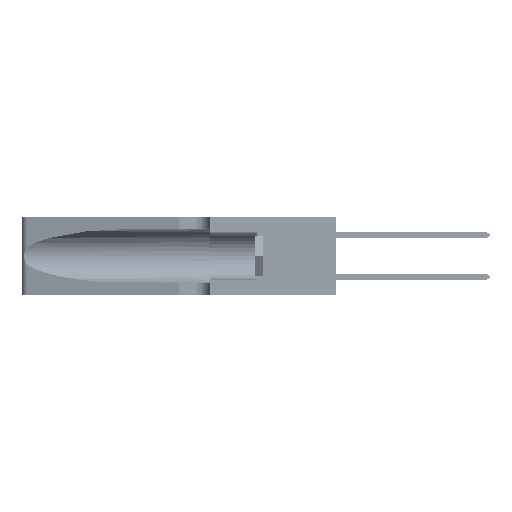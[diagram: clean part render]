
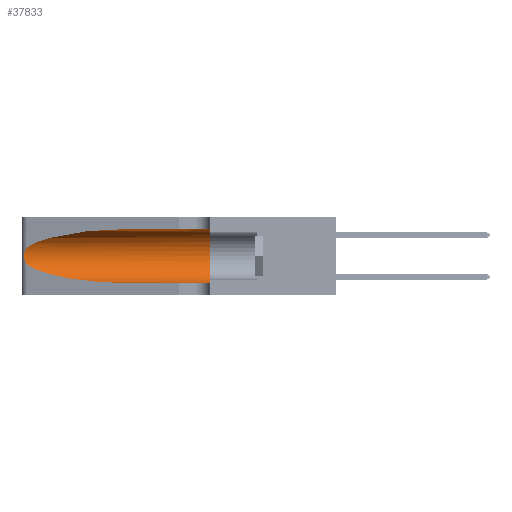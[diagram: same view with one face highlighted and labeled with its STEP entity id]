
A CAD part, left-side view. The second image highlights one B-rep face of the part: STEP entity #37833.
In plain terms, the highlighted cylindrical face has radius 3.308 mm (diameter 6.617 mm), a partial arc.
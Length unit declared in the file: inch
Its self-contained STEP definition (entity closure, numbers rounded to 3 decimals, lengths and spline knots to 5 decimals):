
#127 = CARTESIAN_POINT ( 'NONE',  ( 0.1305, 0.35, 0.185 ) ) ;
#399 = DIRECTION ( 'NONE',  ( 0., 0., -1. ) ) ;
#615 = CARTESIAN_POINT ( 'NONE',  ( 0.25639, 1.23186, 0.15144 ) ) ;
#1072 = ORIENTED_EDGE ( 'NONE', *, *, #36134, .T. ) ;
#2564 = ORIENTED_EDGE ( 'NONE', *, *, #10822, .T. ) ;
#3224 = LINE ( 'NONE', #31769, #21504 ) ;
#4847 = EDGE_LOOP ( 'NONE', ( #1072, #2564, #7027, #9130, #8624, #18576 ) ) ;
#6665 = EDGE_CURVE ( 'NONE', #41783, #29272, #3224, .T. ) ;
#7027 = ORIENTED_EDGE ( 'NONE', *, *, #41073, .T. ) ;
#7701 = CARTESIAN_POINT ( 'NONE',  ( 0.25555, 1.22993, 0.14849 ) ) ;
#7929 = CARTESIAN_POINT ( 'NONE',  ( 0.25487, 1.22718, 0.14631 ) ) ;
#8624 = ORIENTED_EDGE ( 'NONE', *, *, #37200, .F. ) ;
#9105 =( BOUNDED_CURVE ( )  B_SPLINE_CURVE ( 3, ( #7929, #34101, #14827, #41223 ),
 .UNSPECIFIED., .F., .F. ) 
 B_SPLINE_CURVE_WITH_KNOTS ( ( 4, 4 ),
 ( 3.44316, 4.71239 ),
 .UNSPECIFIED. ) 
 CURVE ( )  GEOMETRIC_REPRESENTATION_ITEM ( )  RATIONAL_B_SPLINE_CURVE ( ( 1., 0.87, 0.87, 1. ) ) 
 REPRESENTATION_ITEM ( '' )  );
#9130 = ORIENTED_EDGE ( 'NONE', *, *, #43528, .T. ) ;
#10653 = CARTESIAN_POINT ( 'NONE',  ( 0.25487, 1.22718, 0.22369 ) ) ;
#10822 = EDGE_CURVE ( 'NONE', #26432, #28056, #36006, .T. ) ;
#11378 = FACE_OUTER_BOUND ( 'NONE', #4847, .T. ) ;
#12547 = CYLINDRICAL_SURFACE ( 'NONE', #44460, 0.13025 ) ;
#14827 = CARTESIAN_POINT ( 'NONE',  ( 0.18966, 0.96281, 0.05475 ) ) ;
#15908 = CARTESIAN_POINT ( 'NONE',  ( 0.1305, 0.35, 0.31525 ) ) ;
#16165 = CARTESIAN_POINT ( 'NONE',  ( 0.25487, 1.22718, 0.14631 ) ) ;
#18576 = ORIENTED_EDGE ( 'NONE', *, *, #6665, .F. ) ;
#21504 = VECTOR ( 'NONE', #27485, 39.37008 ) ;
#21630 = VECTOR ( 'NONE', #29426, 39.37008 ) ;
#22163 = CARTESIAN_POINT ( 'NONE',  ( 0.25555, 1.22994, 0.2215 ) ) ;
#22607 = CIRCLE ( 'NONE', #30715, 0.13025 ) ;
#22977 = CARTESIAN_POINT ( 'NONE',  ( 0.25789, 1.23486, 0.15765 ) ) ;
#23130 = CARTESIAN_POINT ( 'NONE',  ( 0.25856, 1.23593, 0.16098 ) ) ;
#24032 = CARTESIAN_POINT ( 'NONE',  ( 0.2373, 1.15595, 0.28018 ) ) ;
#26219 = DIRECTION ( 'NONE',  ( 0., -1., 0. ) ) ;
#26238 = CARTESIAN_POINT ( 'NONE',  ( 0.1305, 0.35, 0.05475 ) ) ;
#26432 = VERTEX_POINT ( 'NONE', #33419 ) ;
#26607 = CARTESIAN_POINT ( 'NONE',  ( 0.26017, 1.23833, 0.17102 ) ) ;
#26736 = DIRECTION ( 'NONE',  ( 0., 0., 1. ) ) ;
#27485 = DIRECTION ( 'NONE',  ( 0., -1., 0. ) ) ;
#28056 = VERTEX_POINT ( 'NONE', #16165 ) ;
#29272 = VERTEX_POINT ( 'NONE', #15908 ) ;
#29426 = DIRECTION ( 'NONE',  ( 0., -1., 0. ) ) ;
#30715 = AXIS2_PLACEMENT_3D ( 'NONE', #127, #48725, #26736 ) ;
#31642 = LINE ( 'NONE', #48757, #21630 ) ;
#31769 = CARTESIAN_POINT ( 'NONE',  ( 0.1305, 1.61858, 0.31525 ) ) ;
#33419 = CARTESIAN_POINT ( 'NONE',  ( 0.25487, 1.22718, 0.22369 ) ) ;
#34101 = CARTESIAN_POINT ( 'NONE',  ( 0.2373, 1.15595, 0.08982 ) ) ;
#34506 = CARTESIAN_POINT ( 'NONE',  ( 0.25487, 1.22718, 0.14631 ) ) ;
#35426 = CARTESIAN_POINT ( 'NONE',  ( 0.25487, 1.22718, 0.22369 ) ) ;
#36006 = B_SPLINE_CURVE_WITH_KNOTS ( 'NONE', 3,
 ( #10653, #22163, #37004, #44639, #48439, #42126, #41477, #45777, #26607, #23130, #22977, #615, #7701, #34506 ),
 .UNSPECIFIED., .F., .F.,
 ( 4, 2, 2, 2, 2, 2, 4 ),
 ( 0., 0.00027, 0.00053, 0.00107, 0.0016, 0.00187, 0.00214 ),
 .UNSPECIFIED. ) ;
#36134 = EDGE_CURVE ( 'NONE', #41783, #26432, #43285, .T. ) ;
#37004 = CARTESIAN_POINT ( 'NONE',  ( 0.25639, 1.23184, 0.21858 ) ) ;
#37200 = EDGE_CURVE ( 'NONE', #29272, #40285, #22607, .T. ) ;
#37833 = ADVANCED_FACE ( 'NONE', ( #11378 ), #12547, .F. ) ;
#38315 = CARTESIAN_POINT ( 'NONE',  ( 0.1305, 0.72297, 0.31525 ) ) ;
#39038 = CARTESIAN_POINT ( 'NONE',  ( 0.1305, 0.72297, 0.31525 ) ) ;
#40285 = VERTEX_POINT ( 'NONE', #26238 ) ;
#41073 = EDGE_CURVE ( 'NONE', #28056, #47740, #9105, .T. ) ;
#41223 = CARTESIAN_POINT ( 'NONE',  ( 0.1305, 0.72297, 0.05475 ) ) ;
#41477 = CARTESIAN_POINT ( 'NONE',  ( 0.26075, 1.23896, 0.19203 ) ) ;
#41783 = VERTEX_POINT ( 'NONE', #38315 ) ;
#42126 = CARTESIAN_POINT ( 'NONE',  ( 0.26018, 1.23835, 0.19895 ) ) ;
#42543 = CARTESIAN_POINT ( 'NONE',  ( 0.1305, 0.72297, 0.05475 ) ) ;
#43285 =( BOUNDED_CURVE ( )  B_SPLINE_CURVE ( 3, ( #39038, #46681, #24032, #35426 ),
 .UNSPECIFIED., .F., .F. ) 
 B_SPLINE_CURVE_WITH_KNOTS ( ( 4, 4 ),
 ( 1.5708, 2.84003 ),
 .UNSPECIFIED. ) 
 CURVE ( )  GEOMETRIC_REPRESENTATION_ITEM ( )  RATIONAL_B_SPLINE_CURVE ( ( 1., 0.87, 0.87, 1. ) ) 
 REPRESENTATION_ITEM ( '' )  );
#43528 = EDGE_CURVE ( 'NONE', #47740, #40285, #31642, .T. ) ;
#44460 = AXIS2_PLACEMENT_3D ( 'NONE', #45563, #26219, #399 ) ;
#44639 = CARTESIAN_POINT ( 'NONE',  ( 0.25787, 1.23484, 0.2124 ) ) ;
#45563 = CARTESIAN_POINT ( 'NONE',  ( 0.1305, 1.61858, 0.185 ) ) ;
#45777 = CARTESIAN_POINT ( 'NONE',  ( 0.26075, 1.23896, 0.178 ) ) ;
#46681 = CARTESIAN_POINT ( 'NONE',  ( 0.18966, 0.96281, 0.31525 ) ) ;
#47740 = VERTEX_POINT ( 'NONE', #42543 ) ;
#48439 = CARTESIAN_POINT ( 'NONE',  ( 0.25854, 1.2359, 0.20912 ) ) ;
#48725 = DIRECTION ( 'NONE',  ( 0., 1., 0. ) ) ;
#48757 = CARTESIAN_POINT ( 'NONE',  ( 0.1305, 1.61858, 0.05475 ) ) ;
